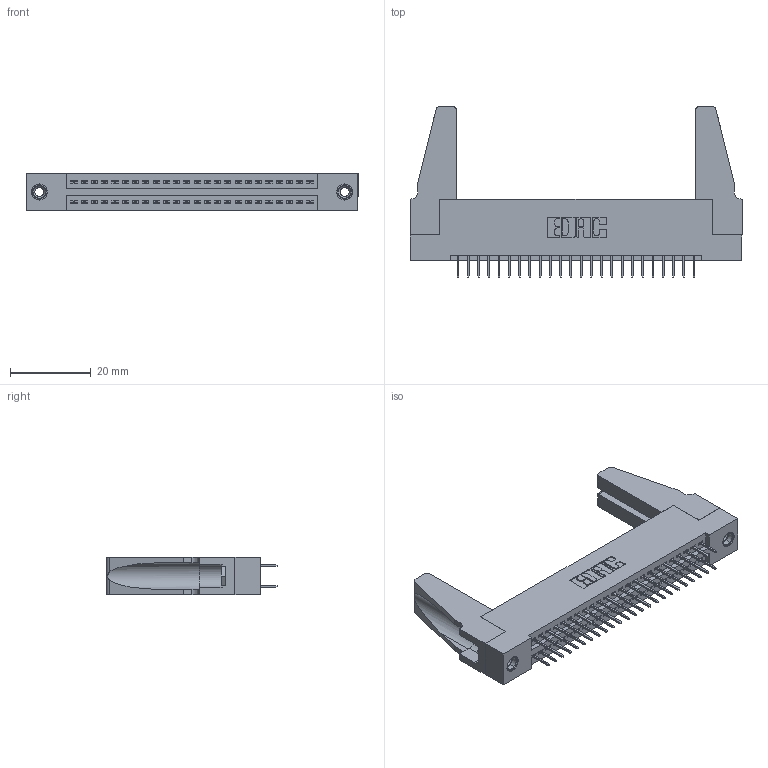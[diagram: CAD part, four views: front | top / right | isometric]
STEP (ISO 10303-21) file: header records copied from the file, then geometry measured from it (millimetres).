
FILE_DESCRIPTION (( 'STEP AP203' ), '1' );
FILE_NAME ('345-048-524-288.STEP', '2019-10-29T04:24:09', ( '' ), ( '' ), 'SwSTEP 2.0', 'SolidWorks 2016', '' );
FILE_SCHEMA (( 'CONFIG_CONTROL_DESIGN' ));
Length unit declared in the file: inch
Products named in the file (5): 345-250-001_345-250-001-102; 345-220-078_345-220-088; 345-048-524-288; 345 Part_Flush Mounting Lugs - 0.156 Dia-TH; 345-292-001_345-293-124
Assembly tree (53 placements, depth 2):
  345-048-524-288
    345 Part_Flush Mounting Lugs - 0.156 Dia-TH
    345-292-001_345-293-124  x48
    345-250-001_345-250-001-102  x2
    345-220-078_345-220-088  x2
Bounding box: 82.19 x 42.21 x 9.4 mm (x, y, z)
Volume: 10997.2 mm3; surface area: 14029.8 mm2
Topology: 53 solids, 53 shells, 2842 faces, 7999 edges, 5130 vertices
Faces by surface type: plane 2024, cylinder 802, cone 12, torus 4
Entity records: 23476 total; most frequent: CARTESIAN_POINT 3946, ORIENTED_EDGE 3840, DIRECTION 3508, EDGE_CURVE 1920, LINE 1654, VECTOR 1654, VERTEX_POINT 1270, AXIS2_PLACEMENT_3D 927
